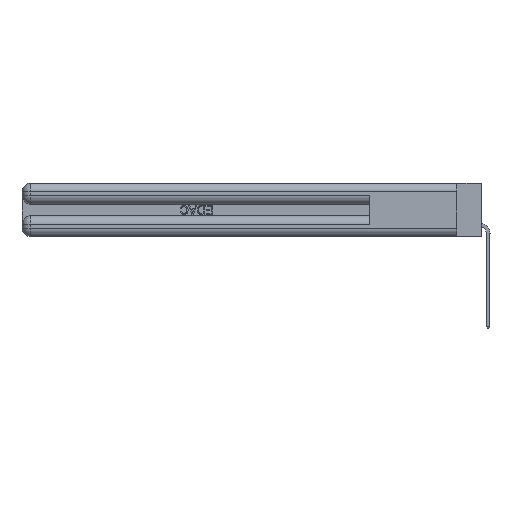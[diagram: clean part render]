
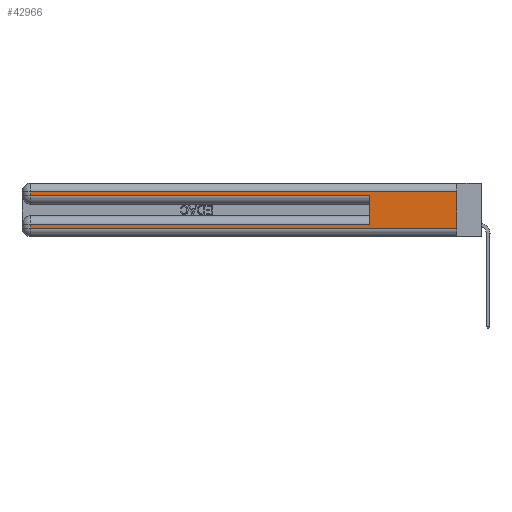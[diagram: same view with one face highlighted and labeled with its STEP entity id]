
A CAD part, left-side view. The second image highlights one B-rep face of the part: STEP entity #42966.
In plain terms, the highlighted planar face has unit normal (-1, 0, 0).
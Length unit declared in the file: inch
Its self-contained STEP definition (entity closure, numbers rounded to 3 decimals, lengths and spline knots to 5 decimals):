
#226 = LINE ( 'NONE', #35394, #36236 ) ;
#1561 = DIRECTION ( 'NONE',  ( 0., -1., 0. ) ) ;
#1727 = CARTESIAN_POINT ( 'NONE',  ( 0., 0., 0.285 ) ) ;
#3603 = EDGE_CURVE ( 'NONE', #42594, #13028, #13189, .T. ) ;
#3928 = ORIENTED_EDGE ( 'NONE', *, *, #40416, .T. ) ;
#4033 = EDGE_CURVE ( 'NONE', #8894, #44142, #39954, .T. ) ;
#5858 = CARTESIAN_POINT ( 'NONE',  ( 0., 0.6, 0.145 ) ) ;
#8894 = VERTEX_POINT ( 'NONE', #32957 ) ;
#9169 = LINE ( 'NONE', #12906, #25622 ) ;
#9202 = ORIENTED_EDGE ( 'NONE', *, *, #25119, .F. ) ;
#10393 = AXIS2_PLACEMENT_3D ( 'NONE', #14096, #41739, #13949 ) ;
#10544 = CARTESIAN_POINT ( 'NONE',  ( 0., 0., 0.06 ) ) ;
#11756 = EDGE_CURVE ( 'NONE', #22126, #46540, #29335, .T. ) ;
#12706 = ORIENTED_EDGE ( 'NONE', *, *, #50275, .T. ) ;
#12906 = CARTESIAN_POINT ( 'NONE',  ( 0., 0., 0.06 ) ) ;
#13028 = VERTEX_POINT ( 'NONE', #10544 ) ;
#13189 = LINE ( 'NONE', #17254, #44919 ) ;
#13331 = CARTESIAN_POINT ( 'NONE',  ( 0., 2.94, 0.06 ) ) ;
#13949 = DIRECTION ( 'NONE',  ( 0., 0., -1. ) ) ;
#14096 = CARTESIAN_POINT ( 'NONE',  ( 0., 0., 0.37 ) ) ;
#16245 = CARTESIAN_POINT ( 'NONE',  ( 0., 2.94, 0.285 ) ) ;
#17254 = CARTESIAN_POINT ( 'NONE',  ( 0., 0., 0.37 ) ) ;
#17466 = CARTESIAN_POINT ( 'NONE',  ( 0., 0.6, 0.285 ) ) ;
#18984 = VECTOR ( 'NONE', #44921, 39.37008 ) ;
#19589 = ORIENTED_EDGE ( 'NONE', *, *, #3603, .F. ) ;
#20068 = CARTESIAN_POINT ( 'NONE',  ( 0., 0.6, 0.085 ) ) ;
#20671 = DIRECTION ( 'NONE',  ( 0., 0., -1. ) ) ;
#21878 = VECTOR ( 'NONE', #45979, 39.37008 ) ;
#22126 = VERTEX_POINT ( 'NONE', #16245 ) ;
#22870 = VECTOR ( 'NONE', #20671, 39.37008 ) ;
#24400 = FACE_OUTER_BOUND ( 'NONE', #37829, .T. ) ;
#25119 = EDGE_CURVE ( 'NONE', #35054, #46540, #33081, .T. ) ;
#25622 = VECTOR ( 'NONE', #32172, 39.37008 ) ;
#26239 = EDGE_CURVE ( 'NONE', #44142, #13028, #9169, .T. ) ;
#29335 = LINE ( 'NONE', #1727, #43969 ) ;
#31769 = CARTESIAN_POINT ( 'NONE',  ( 0., 2.94, 0.37 ) ) ;
#31875 = CARTESIAN_POINT ( 'NONE',  ( 0., 2.94, 0.37 ) ) ;
#32172 = DIRECTION ( 'NONE',  ( 0., -1., 0. ) ) ;
#32957 = CARTESIAN_POINT ( 'NONE',  ( 0., 2.94, 0.085 ) ) ;
#33081 = LINE ( 'NONE', #5858, #18984 ) ;
#35054 = VERTEX_POINT ( 'NONE', #20068 ) ;
#35394 = CARTESIAN_POINT ( 'NONE',  ( 0., 0., 0.31 ) ) ;
#36236 = VECTOR ( 'NONE', #43736, 39.37008 ) ;
#36546 = DIRECTION ( 'NONE',  ( 0., 0., -1. ) ) ;
#37195 = EDGE_CURVE ( 'NONE', #35054, #8894, #42644, .T. ) ;
#37829 = EDGE_LOOP ( 'NONE', ( #19589, #3928, #12706, #40078, #9202, #44925, #42711, #48016 ) ) ;
#39762 = VERTEX_POINT ( 'NONE', #46933 ) ;
#39954 = LINE ( 'NONE', #31769, #22870 ) ;
#40078 = ORIENTED_EDGE ( 'NONE', *, *, #11756, .T. ) ;
#40416 = EDGE_CURVE ( 'NONE', #42594, #39762, #226, .T. ) ;
#41739 = DIRECTION ( 'NONE',  ( 1., 0., 0. ) ) ;
#41872 = CARTESIAN_POINT ( 'NONE',  ( 0., 0., 0.085 ) ) ;
#42594 = VERTEX_POINT ( 'NONE', #46928 ) ;
#42644 = LINE ( 'NONE', #41872, #21878 ) ;
#42711 = ORIENTED_EDGE ( 'NONE', *, *, #4033, .T. ) ;
#42966 = ADVANCED_FACE ( 'NONE', ( #24400 ), #44668, .F. ) ;
#43736 = DIRECTION ( 'NONE',  ( 0., 1., 0. ) ) ;
#43969 = VECTOR ( 'NONE', #1561, 39.37008 ) ;
#44142 = VERTEX_POINT ( 'NONE', #13331 ) ;
#44668 = PLANE ( 'NONE',  #10393 ) ;
#44919 = VECTOR ( 'NONE', #36546, 39.37008 ) ;
#44921 = DIRECTION ( 'NONE',  ( 0., 0., 1. ) ) ;
#44925 = ORIENTED_EDGE ( 'NONE', *, *, #37195, .T. ) ;
#45979 = DIRECTION ( 'NONE',  ( 0., 1., 0. ) ) ;
#46540 = VERTEX_POINT ( 'NONE', #17466 ) ;
#46928 = CARTESIAN_POINT ( 'NONE',  ( 0., 0., 0.31 ) ) ;
#46933 = CARTESIAN_POINT ( 'NONE',  ( 0., 2.94, 0.31 ) ) ;
#47287 = DIRECTION ( 'NONE',  ( 0., 0., -1. ) ) ;
#47332 = VECTOR ( 'NONE', #47287, 39.37008 ) ;
#48016 = ORIENTED_EDGE ( 'NONE', *, *, #26239, .T. ) ;
#48578 = LINE ( 'NONE', #31875, #47332 ) ;
#50275 = EDGE_CURVE ( 'NONE', #39762, #22126, #48578, .T. ) ;
